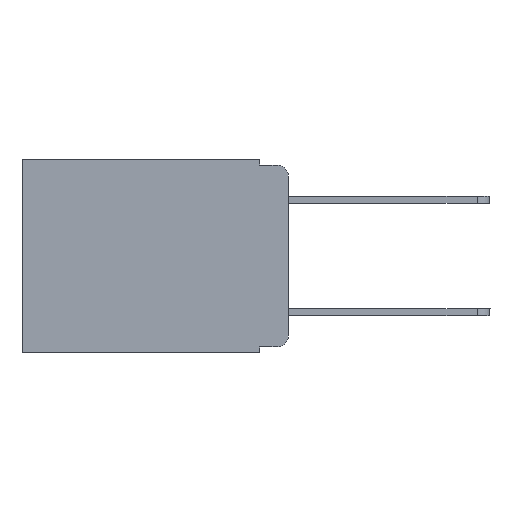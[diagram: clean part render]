
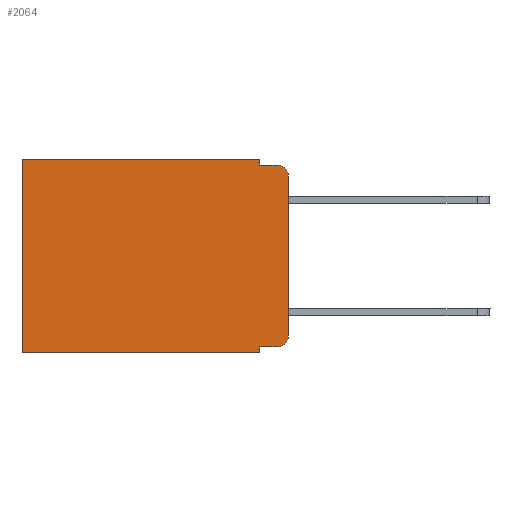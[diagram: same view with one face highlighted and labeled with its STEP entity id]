
A CAD part, left-side view. The second image highlights one B-rep face of the part: STEP entity #2064.
In plain terms, the highlighted planar face has unit normal (-1, 0, 0).
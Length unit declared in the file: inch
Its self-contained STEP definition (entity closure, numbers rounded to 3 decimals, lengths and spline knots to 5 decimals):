
#109 = VECTOR ( 'NONE', #15207, 39.37008 ) ;
#242 = EDGE_LOOP ( 'NONE', ( #2481, #14392, #1968, #3850, #2783, #8600, #3711, #1334, #2390, #14584 ) ) ;
#410 = DIRECTION ( 'NONE',  ( 0., 0., -1. ) ) ;
#501 = CARTESIAN_POINT ( 'NONE',  ( 0.298, 0., -0.03 ) ) ;
#685 = DIRECTION ( 'NONE',  ( 0., 0., -1. ) ) ;
#1049 = DIRECTION ( 'NONE',  ( 0., 1., 0. ) ) ;
#1182 = DIRECTION ( 'NONE',  ( 0., 1., 0. ) ) ;
#1334 = ORIENTED_EDGE ( 'NONE', *, *, #14449, .F. ) ;
#1376 = CARTESIAN_POINT ( 'NONE',  ( 0.298, 0.051, 0. ) ) ;
#1870 = AXIS2_PLACEMENT_3D ( 'NONE', #1954, #11619, #685 ) ;
#1954 = CARTESIAN_POINT ( 'NONE',  ( 0.298, 0.02, -0.313 ) ) ;
#1968 = ORIENTED_EDGE ( 'NONE', *, *, #11970, .F. ) ;
#2064 = ADVANCED_FACE ( 'NONE', ( #14220 ), #3321, .F. ) ;
#2163 = CIRCLE ( 'NONE', #1870, 0.02 ) ;
#2251 = LINE ( 'NONE', #3079, #12405 ) ;
#2390 = ORIENTED_EDGE ( 'NONE', *, *, #6104, .T. ) ;
#2430 = VERTEX_POINT ( 'NONE', #11552 ) ;
#2481 = ORIENTED_EDGE ( 'NONE', *, *, #11180, .F. ) ;
#2501 = VECTOR ( 'NONE', #4240, 39.37008 ) ;
#2783 = ORIENTED_EDGE ( 'NONE', *, *, #3069, .T. ) ;
#3069 = EDGE_CURVE ( 'NONE', #11498, #10703, #14001, .T. ) ;
#3079 = CARTESIAN_POINT ( 'NONE',  ( 0.298, 0.051, -0.333 ) ) ;
#3321 = PLANE ( 'NONE',  #6954 ) ;
#3371 = CARTESIAN_POINT ( 'NONE',  ( 0.298, 0.051, 0. ) ) ;
#3375 = DIRECTION ( 'NONE',  ( 0., 0., -1. ) ) ;
#3711 = ORIENTED_EDGE ( 'NONE', *, *, #8239, .F. ) ;
#3850 = ORIENTED_EDGE ( 'NONE', *, *, #8958, .F. ) ;
#4152 = CARTESIAN_POINT ( 'NONE',  ( 0.298, 0., 0. ) ) ;
#4240 = DIRECTION ( 'NONE',  ( 0., 0., -1. ) ) ;
#4345 = CARTESIAN_POINT ( 'NONE',  ( 0.298, 0.473, 0. ) ) ;
#4530 = VERTEX_POINT ( 'NONE', #501 ) ;
#5314 = VERTEX_POINT ( 'NONE', #13017 ) ;
#5370 = DIRECTION ( 'NONE',  ( 0., 0., -1. ) ) ;
#5556 = VECTOR ( 'NONE', #410, 39.37008 ) ;
#5589 = CARTESIAN_POINT ( 'NONE',  ( 0.298, 0.051, -0.01 ) ) ;
#6104 = EDGE_CURVE ( 'NONE', #15189, #10996, #2251, .T. ) ;
#6293 = CARTESIAN_POINT ( 'NONE',  ( 0.298, 0.02, -0.03 ) ) ;
#6400 = CARTESIAN_POINT ( 'NONE',  ( 0.298, 0.473, 0. ) ) ;
#6634 = AXIS2_PLACEMENT_3D ( 'NONE', #6293, #14711, #9936 ) ;
#6688 = CARTESIAN_POINT ( 'NONE',  ( 0.298, 0.473, -0.343 ) ) ;
#6726 = LINE ( 'NONE', #5589, #109 ) ;
#6893 = CARTESIAN_POINT ( 'NONE',  ( 0.298, 0.051, -0.343 ) ) ;
#6937 = DIRECTION ( 'NONE',  ( 0., 0., -1. ) ) ;
#6954 = AXIS2_PLACEMENT_3D ( 'NONE', #9305, #8291, #3375 ) ;
#7047 = LINE ( 'NONE', #4345, #2501 ) ;
#8239 = EDGE_CURVE ( 'NONE', #13319, #14308, #12144, .T. ) ;
#8291 = DIRECTION ( 'NONE',  ( 1., 0., 0. ) ) ;
#8385 = LINE ( 'NONE', #1376, #5556 ) ;
#8600 = ORIENTED_EDGE ( 'NONE', *, *, #14298, .T. ) ;
#8741 = VECTOR ( 'NONE', #1049, 39.37008 ) ;
#8958 = EDGE_CURVE ( 'NONE', #11498, #13357, #8385, .T. ) ;
#9054 = DIRECTION ( 'NONE',  ( 0., -1., 0. ) ) ;
#9075 = EDGE_CURVE ( 'NONE', #10996, #5314, #2163, .T. ) ;
#9305 = CARTESIAN_POINT ( 'NONE',  ( 0.298, 0., 0. ) ) ;
#9499 = LINE ( 'NONE', #3371, #12471 ) ;
#9610 = EDGE_CURVE ( 'NONE', #4530, #2430, #12101, .T. ) ;
#9643 = VECTOR ( 'NONE', #5370, 39.37008 ) ;
#9936 = DIRECTION ( 'NONE',  ( 0., 0., -1. ) ) ;
#10383 = LINE ( 'NONE', #4152, #9643 ) ;
#10703 = VERTEX_POINT ( 'NONE', #6400 ) ;
#10764 = CARTESIAN_POINT ( 'NONE',  ( 0.298, 0., -0.343 ) ) ;
#10980 = CARTESIAN_POINT ( 'NONE',  ( 0.298, 0.051, 0. ) ) ;
#10996 = VERTEX_POINT ( 'NONE', #13111 ) ;
#11180 = EDGE_CURVE ( 'NONE', #4530, #5314, #10383, .T. ) ;
#11498 = VERTEX_POINT ( 'NONE', #10980 ) ;
#11552 = CARTESIAN_POINT ( 'NONE',  ( 0.298, 0.02, -0.01 ) ) ;
#11619 = DIRECTION ( 'NONE',  ( -1., 0., 0. ) ) ;
#11969 = VECTOR ( 'NONE', #1182, 39.37008 ) ;
#11970 = EDGE_CURVE ( 'NONE', #13357, #2430, #6726, .T. ) ;
#12101 = CIRCLE ( 'NONE', #6634, 0.02 ) ;
#12144 = LINE ( 'NONE', #10764, #11969 ) ;
#12405 = VECTOR ( 'NONE', #9054, 39.37008 ) ;
#12471 = VECTOR ( 'NONE', #6937, 39.37008 ) ;
#13017 = CARTESIAN_POINT ( 'NONE',  ( 0.298, 0., -0.313 ) ) ;
#13111 = CARTESIAN_POINT ( 'NONE',  ( 0.298, 0.02, -0.333 ) ) ;
#13319 = VERTEX_POINT ( 'NONE', #6893 ) ;
#13357 = VERTEX_POINT ( 'NONE', #14133 ) ;
#14001 = LINE ( 'NONE', #14244, #8741 ) ;
#14133 = CARTESIAN_POINT ( 'NONE',  ( 0.298, 0.051, -0.01 ) ) ;
#14220 = FACE_OUTER_BOUND ( 'NONE', #242, .T. ) ;
#14244 = CARTESIAN_POINT ( 'NONE',  ( 0.298, 0., 0. ) ) ;
#14298 = EDGE_CURVE ( 'NONE', #10703, #14308, #7047, .T. ) ;
#14308 = VERTEX_POINT ( 'NONE', #6688 ) ;
#14392 = ORIENTED_EDGE ( 'NONE', *, *, #9610, .T. ) ;
#14421 = CARTESIAN_POINT ( 'NONE',  ( 0.298, 0.051, -0.333 ) ) ;
#14449 = EDGE_CURVE ( 'NONE', #15189, #13319, #9499, .T. ) ;
#14584 = ORIENTED_EDGE ( 'NONE', *, *, #9075, .T. ) ;
#14711 = DIRECTION ( 'NONE',  ( -1., 0., 0. ) ) ;
#15189 = VERTEX_POINT ( 'NONE', #14421 ) ;
#15207 = DIRECTION ( 'NONE',  ( 0., -1., 0. ) ) ;
